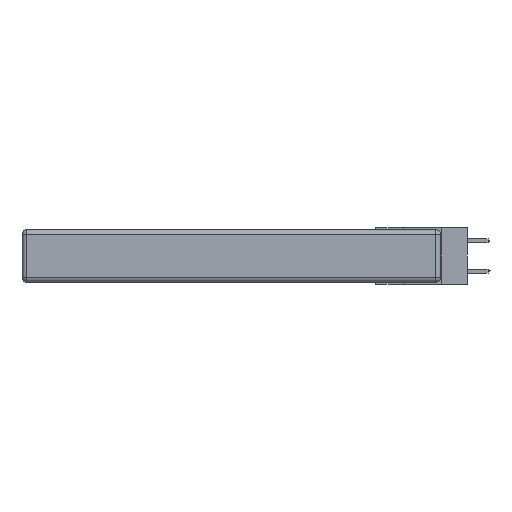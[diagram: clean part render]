
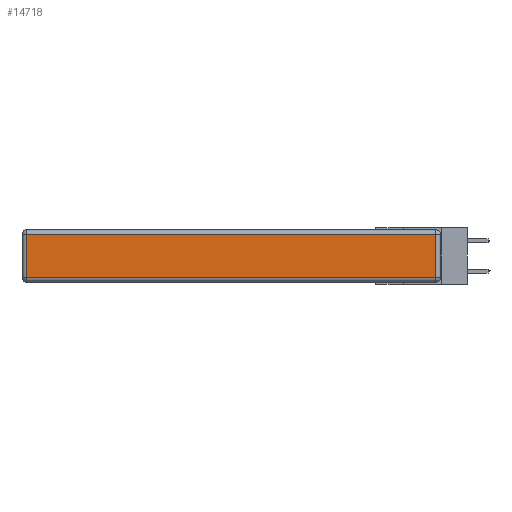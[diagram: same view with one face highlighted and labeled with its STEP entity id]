
A CAD part, left-side view. The second image highlights one B-rep face of the part: STEP entity #14718.
In plain terms, the highlighted planar face has unit normal (-1, 0, 0).
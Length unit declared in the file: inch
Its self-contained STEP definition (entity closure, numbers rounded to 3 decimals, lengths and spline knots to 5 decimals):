
#713 = FACE_OUTER_BOUND ( 'NONE', #1366, .T. ) ;
#792 = CARTESIAN_POINT ( 'NONE',  ( 0., 2.75, -0.03 ) ) ;
#865 = CARTESIAN_POINT ( 'NONE',  ( 0., 0., -0.343 ) ) ;
#1292 = CARTESIAN_POINT ( 'NONE',  ( 0., 0.03, -0.313 ) ) ;
#1366 = EDGE_LOOP ( 'NONE', ( #3785, #11136, #5716, #6675 ) ) ;
#1959 = DIRECTION ( 'NONE',  ( -1., 0., 0. ) ) ;
#3093 = DIRECTION ( 'NONE',  ( 0., -1., 0. ) ) ;
#3785 = ORIENTED_EDGE ( 'NONE', *, *, #13721, .T. ) ;
#3995 = CARTESIAN_POINT ( 'NONE',  ( 0., 2.72, -0.03 ) ) ;
#5065 = LINE ( 'NONE', #792, #7884 ) ;
#5446 = CARTESIAN_POINT ( 'NONE',  ( 0., 0.03, -0.343 ) ) ;
#5557 = DIRECTION ( 'NONE',  ( 0., 0., -1. ) ) ;
#5716 = ORIENTED_EDGE ( 'NONE', *, *, #13166, .T. ) ;
#6675 = ORIENTED_EDGE ( 'NONE', *, *, #8839, .T. ) ;
#6775 = DIRECTION ( 'NONE',  ( 0., 1., 0. ) ) ;
#7116 = VERTEX_POINT ( 'NONE', #7553 ) ;
#7455 = VECTOR ( 'NONE', #13960, 39.37008 ) ;
#7553 = CARTESIAN_POINT ( 'NONE',  ( 0., 2.72, -0.313 ) ) ;
#7884 = VECTOR ( 'NONE', #6775, 39.37008 ) ;
#7942 = VERTEX_POINT ( 'NONE', #9349 ) ;
#8839 = EDGE_CURVE ( 'NONE', #13696, #7116, #14729, .T. ) ;
#9349 = CARTESIAN_POINT ( 'NONE',  ( 0., 0.03, -0.03 ) ) ;
#10440 = CARTESIAN_POINT ( 'NONE',  ( 0., 2.72, -0.343 ) ) ;
#11136 = ORIENTED_EDGE ( 'NONE', *, *, #14736, .T. ) ;
#11980 = VECTOR ( 'NONE', #3093, 39.37008 ) ;
#12607 = DIRECTION ( 'NONE',  ( 0., 0., 1. ) ) ;
#12629 = AXIS2_PLACEMENT_3D ( 'NONE', #865, #1959, #12607 ) ;
#12671 = VECTOR ( 'NONE', #5557, 39.37008 ) ;
#13166 = EDGE_CURVE ( 'NONE', #7942, #13696, #5065, .T. ) ;
#13696 = VERTEX_POINT ( 'NONE', #3995 ) ;
#13721 = EDGE_CURVE ( 'NONE', #7116, #15025, #15144, .T. ) ;
#13897 = CARTESIAN_POINT ( 'NONE',  ( 0., 0., -0.313 ) ) ;
#13960 = DIRECTION ( 'NONE',  ( 0., 0., 1. ) ) ;
#14718 = ADVANCED_FACE ( 'NONE', ( #713 ), #15027, .T. ) ;
#14726 = LINE ( 'NONE', #5446, #7455 ) ;
#14729 = LINE ( 'NONE', #10440, #12671 ) ;
#14736 = EDGE_CURVE ( 'NONE', #15025, #7942, #14726, .T. ) ;
#15025 = VERTEX_POINT ( 'NONE', #1292 ) ;
#15027 = PLANE ( 'NONE',  #12629 ) ;
#15144 = LINE ( 'NONE', #13897, #11980 ) ;
